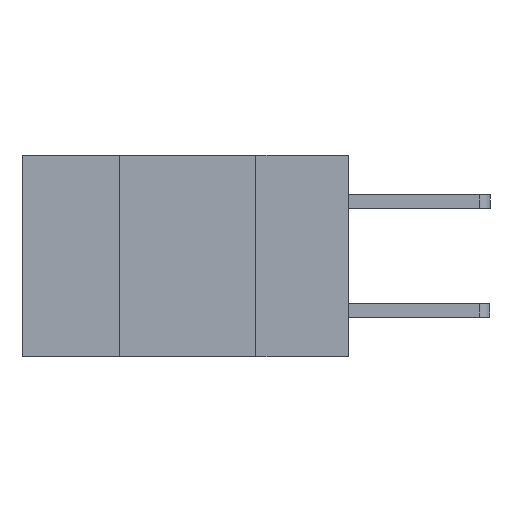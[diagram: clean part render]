
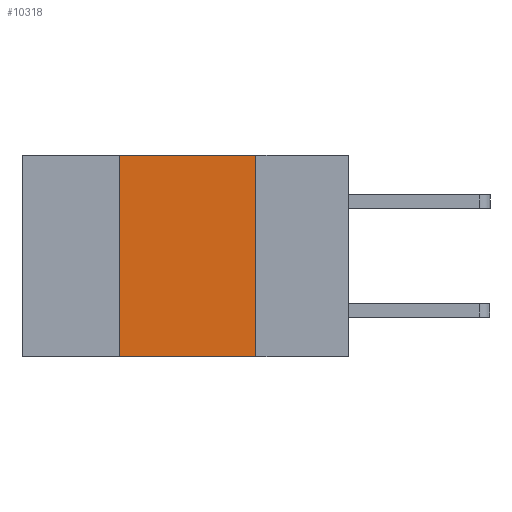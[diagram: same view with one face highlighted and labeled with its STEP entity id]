
A CAD part, left-side view. The second image highlights one B-rep face of the part: STEP entity #10318.
In plain terms, the highlighted planar face has unit normal (-1, 0, 0).
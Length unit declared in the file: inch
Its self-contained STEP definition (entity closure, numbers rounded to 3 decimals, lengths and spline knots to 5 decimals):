
#44 = EDGE_CURVE ( 'NONE', #9585, #2020, #9704, .T. ) ;
#391 = CARTESIAN_POINT ( 'NONE',  ( 0., 0.42, 0. ) ) ;
#778 = VECTOR ( 'NONE', #1542, 39.37008 ) ;
#942 = FACE_OUTER_BOUND ( 'NONE', #3958, .T. ) ;
#1542 = DIRECTION ( 'NONE',  ( 0., 0., -1. ) ) ;
#1814 = EDGE_CURVE ( 'NONE', #3572, #7455, #2993, .T. ) ;
#2020 = VERTEX_POINT ( 'NONE', #9347 ) ;
#2086 = CARTESIAN_POINT ( 'NONE',  ( 0., 0.17, -0.37 ) ) ;
#2496 = DIRECTION ( 'NONE',  ( 0., 0., -1. ) ) ;
#2993 = LINE ( 'NONE', #5846, #778 ) ;
#3572 = VERTEX_POINT ( 'NONE', #10485 ) ;
#3958 = EDGE_LOOP ( 'NONE', ( #10120, #9617, #9872, #5679 ) ) ;
#4025 = LINE ( 'NONE', #7563, #5991 ) ;
#4196 = CARTESIAN_POINT ( 'NONE',  ( 0., 0.6, 0. ) ) ;
#4296 = DIRECTION ( 'NONE',  ( 0., -1., 0. ) ) ;
#4994 = CARTESIAN_POINT ( 'NONE',  ( 0., 0.6, 0. ) ) ;
#5563 = DIRECTION ( 'NONE',  ( 0., 0., 1. ) ) ;
#5679 = ORIENTED_EDGE ( 'NONE', *, *, #6080, .T. ) ;
#5846 = CARTESIAN_POINT ( 'NONE',  ( 0., 0.17, 0. ) ) ;
#5991 = VECTOR ( 'NONE', #4296, 39.37008 ) ;
#6009 = EDGE_CURVE ( 'NONE', #2020, #3572, #8607, .T. ) ;
#6080 = EDGE_CURVE ( 'NONE', #9585, #7455, #4025, .T. ) ;
#6438 = CARTESIAN_POINT ( 'NONE',  ( 0., 0.42, -0.37 ) ) ;
#6487 = VECTOR ( 'NONE', #9044, 39.37008 ) ;
#7385 = PLANE ( 'NONE',  #10188 ) ;
#7423 = DIRECTION ( 'NONE',  ( 1., 0., 0. ) ) ;
#7455 = VERTEX_POINT ( 'NONE', #2086 ) ;
#7563 = CARTESIAN_POINT ( 'NONE',  ( 0., 0.6, -0.37 ) ) ;
#7652 = VECTOR ( 'NONE', #5563, 39.37008 ) ;
#8607 = LINE ( 'NONE', #4196, #6487 ) ;
#9044 = DIRECTION ( 'NONE',  ( 0., -1., 0. ) ) ;
#9347 = CARTESIAN_POINT ( 'NONE',  ( 0., 0.42, 0. ) ) ;
#9585 = VERTEX_POINT ( 'NONE', #6438 ) ;
#9617 = ORIENTED_EDGE ( 'NONE', *, *, #6009, .F. ) ;
#9704 = LINE ( 'NONE', #391, #7652 ) ;
#9872 = ORIENTED_EDGE ( 'NONE', *, *, #44, .F. ) ;
#10120 = ORIENTED_EDGE ( 'NONE', *, *, #1814, .F. ) ;
#10188 = AXIS2_PLACEMENT_3D ( 'NONE', #4994, #7423, #2496 ) ;
#10318 = ADVANCED_FACE ( 'NONE', ( #942 ), #7385, .F. ) ;
#10485 = CARTESIAN_POINT ( 'NONE',  ( 0., 0.17, 0. ) ) ;
